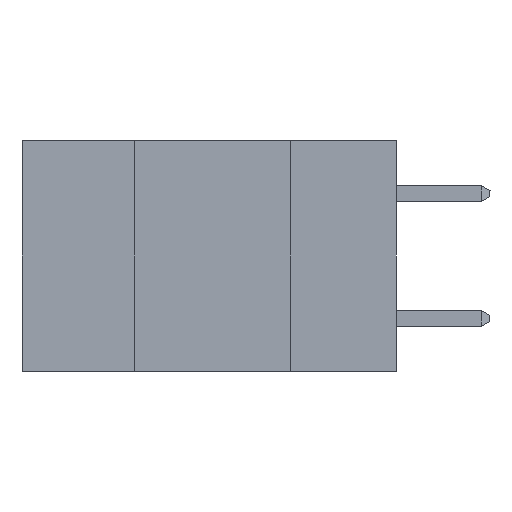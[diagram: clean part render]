
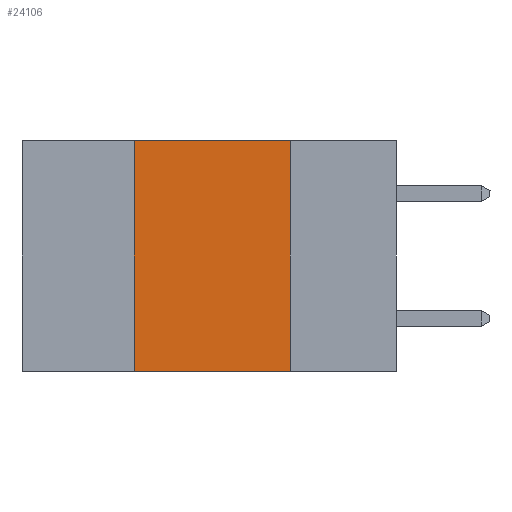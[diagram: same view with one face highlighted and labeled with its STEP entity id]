
A CAD part, left-side view. The second image highlights one B-rep face of the part: STEP entity #24106.
In plain terms, the highlighted planar face has unit normal (-1, 0, 0).
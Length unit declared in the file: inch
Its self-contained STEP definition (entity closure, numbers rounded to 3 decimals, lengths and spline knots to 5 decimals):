
#1499 = PLANE ( 'NONE',  #6567 ) ;
#3168 = ORIENTED_EDGE ( 'NONE', *, *, #14114, .F. ) ;
#3346 = EDGE_CURVE ( 'NONE', #26126, #24238, #23915, .T. ) ;
#3347 = VECTOR ( 'NONE', #24715, 39.37008 ) ;
#3894 = DIRECTION ( 'NONE',  ( 0., 0., -1. ) ) ;
#5129 = DIRECTION ( 'NONE',  ( 0., 0., -1. ) ) ;
#6384 = VERTEX_POINT ( 'NONE', #24343 ) ;
#6567 = AXIS2_PLACEMENT_3D ( 'NONE', #24703, #17814, #3894 ) ;
#11241 = CARTESIAN_POINT ( 'NONE',  ( 0., 0.6, 0. ) ) ;
#11769 = LINE ( 'NONE', #23687, #23324 ) ;
#12388 = CARTESIAN_POINT ( 'NONE',  ( 0., 0.6, -0.37 ) ) ;
#13558 = DIRECTION ( 'NONE',  ( 0., -1., 0. ) ) ;
#13870 = EDGE_CURVE ( 'NONE', #19715, #6384, #28407, .T. ) ;
#14114 = EDGE_CURVE ( 'NONE', #19715, #26126, #21228, .T. ) ;
#14678 = DIRECTION ( 'NONE',  ( 0., -1., 0. ) ) ;
#17612 = EDGE_CURVE ( 'NONE', #24238, #6384, #11769, .T. ) ;
#17814 = DIRECTION ( 'NONE',  ( 1., 0., 0. ) ) ;
#18217 = CARTESIAN_POINT ( 'NONE',  ( 0., 0.17, 0. ) ) ;
#18230 = FACE_OUTER_BOUND ( 'NONE', #22437, .T. ) ;
#18487 = VECTOR ( 'NONE', #13558, 39.37008 ) ;
#19715 = VERTEX_POINT ( 'NONE', #28622 ) ;
#20083 = CARTESIAN_POINT ( 'NONE',  ( 0., 0.42, 0. ) ) ;
#20210 = ORIENTED_EDGE ( 'NONE', *, *, #13870, .T. ) ;
#21228 = LINE ( 'NONE', #20083, #3347 ) ;
#22437 = EDGE_LOOP ( 'NONE', ( #25462, #23506, #3168, #20210 ) ) ;
#22667 = CARTESIAN_POINT ( 'NONE',  ( 0., 0.42, 0. ) ) ;
#23324 = VECTOR ( 'NONE', #5129, 39.37008 ) ;
#23506 = ORIENTED_EDGE ( 'NONE', *, *, #3346, .F. ) ;
#23687 = CARTESIAN_POINT ( 'NONE',  ( 0., 0.17, 0. ) ) ;
#23915 = LINE ( 'NONE', #11241, #18487 ) ;
#24106 = ADVANCED_FACE ( 'NONE', ( #18230 ), #1499, .F. ) ;
#24238 = VERTEX_POINT ( 'NONE', #18217 ) ;
#24343 = CARTESIAN_POINT ( 'NONE',  ( 0., 0.17, -0.37 ) ) ;
#24703 = CARTESIAN_POINT ( 'NONE',  ( 0., 0.6, 0. ) ) ;
#24715 = DIRECTION ( 'NONE',  ( 0., 0., 1. ) ) ;
#25462 = ORIENTED_EDGE ( 'NONE', *, *, #17612, .F. ) ;
#26126 = VERTEX_POINT ( 'NONE', #22667 ) ;
#26965 = VECTOR ( 'NONE', #14678, 39.37008 ) ;
#28407 = LINE ( 'NONE', #12388, #26965 ) ;
#28622 = CARTESIAN_POINT ( 'NONE',  ( 0., 0.42, -0.37 ) ) ;
